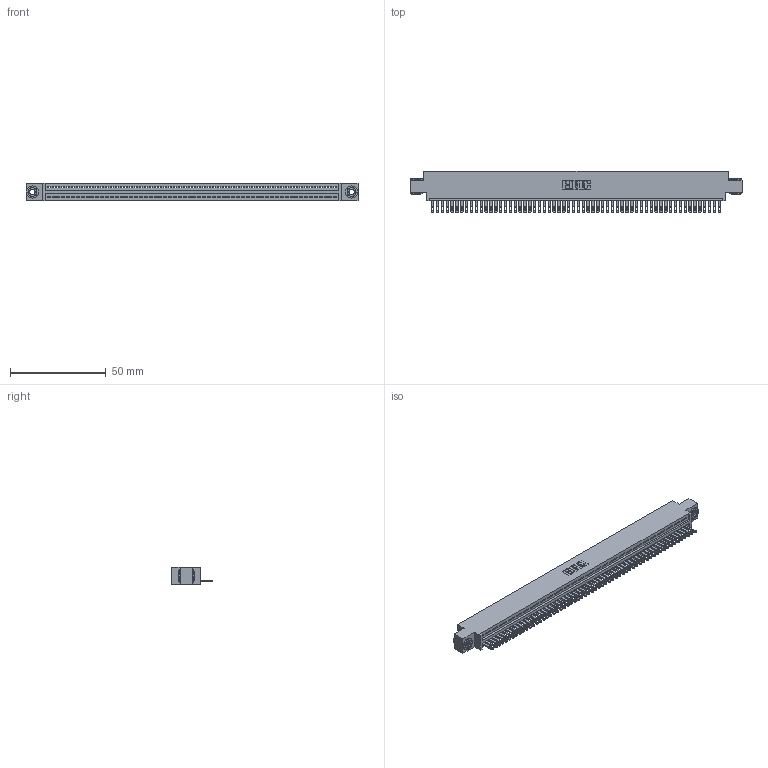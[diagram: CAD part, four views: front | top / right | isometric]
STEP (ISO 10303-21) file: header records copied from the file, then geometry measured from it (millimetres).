
FILE_DESCRIPTION (( 'STEP AP203' ), '1' );
FILE_NAME ('345-060-500-603.STEP', '2018-09-26T22:33:12', ( '' ), ( '' ), 'SwSTEP 2.0', 'SolidWorks 2016', '' );
FILE_SCHEMA (( 'CONFIG_CONTROL_DESIGN' ));
Length unit declared in the file: inch
Products named in the file (4): 345-250-002_345-250-002-102; 345-292-001_345-293-100; 345 Part_0.170 Offset - 0.156 Dia-TH; 345-060-500-603
Assembly tree (63 placements, depth 2):
  345-060-500-603
    345 Part_0.170 Offset - 0.156 Dia-TH
    345-292-001_345-293-100  x60
    345-250-002_345-250-002-102  x2
Bounding box: 173.61 x 21.51 x 9.4 mm (x, y, z)
Volume: 16580.2 mm3; surface area: 22753.9 mm2
Topology: 63 solids, 63 shells, 3408 faces, 10509 edges, 7002 vertices
Faces by surface type: plane 2134, cylinder 1266, cone 8
Entity records: 43446 total; most frequent: CARTESIAN_POINT 7503, ORIENTED_EDGE 7490, DIRECTION 6559, EDGE_CURVE 3745, VECTOR 3345, LINE 3345, VERTEX_POINT 2494, AXIS2_PLACEMENT_3D 1607
